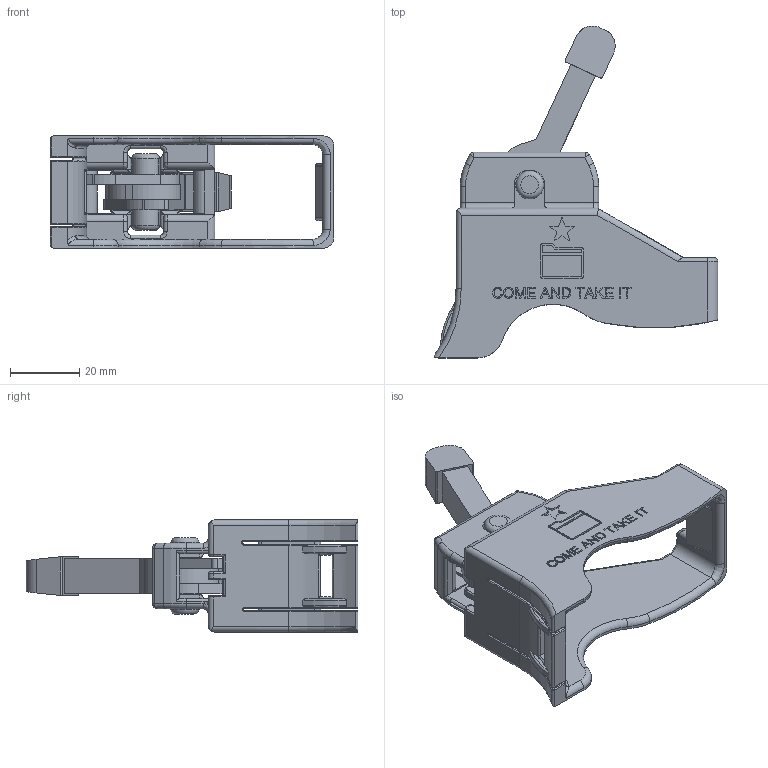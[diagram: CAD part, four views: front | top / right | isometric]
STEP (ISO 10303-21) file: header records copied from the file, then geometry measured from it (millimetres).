
FILE_DESCRIPTION(/* description */ (''),/* implementation_level */ '2;1');
FILE_NAME(/* name */ 'freeman1337_freeloader-AK-edition_all.step',/* time_stamp */ '2021-12-15T20:55:55-08:00',/* author */ (''),/* organization */ (''),/* preprocessor_version */ 'ST-DEVELOPER v18.1',/* originating_system */ 'Autodesk Translation Framework v10.10.0.1391',/* authorisation */ '');
FILE_SCHEMA (('AUTOMOTIVE_DESIGN { 1 0 10303 214 3 1 1 }'));
Products named in the file (1): (Unsaved)
Bounding box: 82.1 x 96 x 32.45 mm (x, y, z)
Volume: 32374.2 mm3; surface area: 22145.3 mm2
Topology: 2 solids, 2 shells, 1567 faces, 4237 edges, 2763 vertices
Faces by surface type: plane 786, bspline 499, cylinder 213, torus 69
Entity records: 54170 total; most frequent: CARTESIAN_POINT 18212, ORIENTED_EDGE 8454, DIRECTION 5836, EDGE_CURVE 4227, VERTEX_POINT 2763, LINE 2652, VECTOR 2652, EDGE_LOOP 1680
